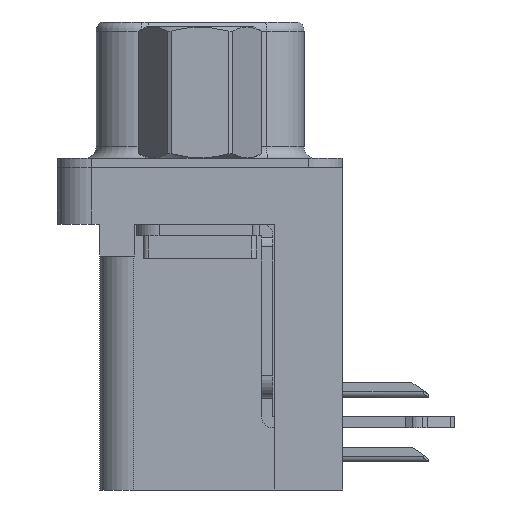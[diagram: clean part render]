
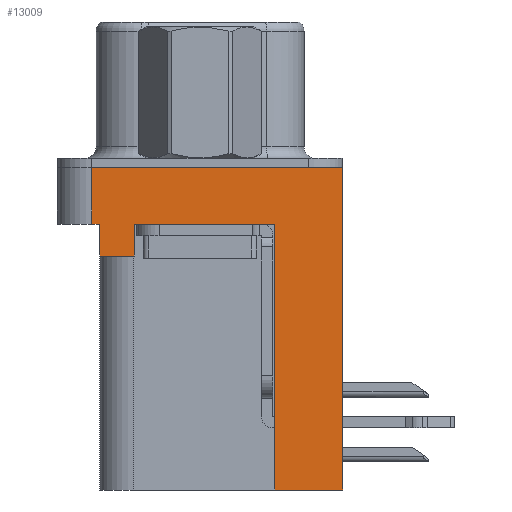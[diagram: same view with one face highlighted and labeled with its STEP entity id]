
A CAD part, left-side view. The second image highlights one B-rep face of the part: STEP entity #13009.
In plain terms, the highlighted planar face has unit normal (-1, 0, 0).
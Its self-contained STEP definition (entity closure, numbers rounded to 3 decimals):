
#144 = DIRECTION ( 'NONE',  ( 0., 1., 0. ) ) ;
#608 = CARTESIAN_POINT ( 'NONE',  ( -2.935, -6.275, -2.5 ) ) ;
#671 = VERTEX_POINT ( 'NONE', #20558 ) ;
#675 = VECTOR ( 'NONE', #144, 1000. ) ;
#1145 = CARTESIAN_POINT ( 'NONE',  ( -2.935, -6.275, 0. ) ) ;
#1560 = ORIENTED_EDGE ( 'NONE', *, *, #6238, .T. ) ;
#1581 = DIRECTION ( 'NONE',  ( 0., 0., 1. ) ) ;
#1715 = VERTEX_POINT ( 'NONE', #3816 ) ;
#1782 = CARTESIAN_POINT ( 'NONE',  ( -2.935, -6.275, -2.5 ) ) ;
#1913 = DIRECTION ( 'NONE',  ( 0., 0., 1. ) ) ;
#2252 = LINE ( 'NONE', #1782, #15737 ) ;
#2701 = EDGE_CURVE ( 'NONE', #4953, #7491, #7472, .T. ) ;
#2882 = VECTOR ( 'NONE', #22540, 1000. ) ;
#3191 = VERTEX_POINT ( 'NONE', #9280 ) ;
#3260 = DIRECTION ( 'NONE',  ( -1., 0., 0. ) ) ;
#3447 = DIRECTION ( 'NONE',  ( 0., 1., 0. ) ) ;
#3816 = CARTESIAN_POINT ( 'NONE',  ( -2.935, 2.895, -3.9 ) ) ;
#4017 = VECTOR ( 'NONE', #13824, 1000. ) ;
#4367 = VERTEX_POINT ( 'NONE', #1145 ) ;
#4953 = VERTEX_POINT ( 'NONE', #17877 ) ;
#5112 = FACE_OUTER_BOUND ( 'NONE', #14673, .T. ) ;
#5214 = LINE ( 'NONE', #7188, #12640 ) ;
#5245 = VERTEX_POINT ( 'NONE', #13289 ) ;
#5697 = ORIENTED_EDGE ( 'NONE', *, *, #7533, .F. ) ;
#6238 = EDGE_CURVE ( 'NONE', #671, #11153, #6294, .T. ) ;
#6294 = LINE ( 'NONE', #608, #4017 ) ;
#6390 = VECTOR ( 'NONE', #9056, 1000. ) ;
#6643 = LINE ( 'NONE', #15786, #23286 ) ;
#7016 = CARTESIAN_POINT ( 'NONE',  ( -2.935, 4.425, -2.5 ) ) ;
#7090 = CARTESIAN_POINT ( 'NONE',  ( -2.935, 4.425, -3.9 ) ) ;
#7188 = CARTESIAN_POINT ( 'NONE',  ( -2.935, -6.275, 0. ) ) ;
#7472 = LINE ( 'NONE', #15000, #2882 ) ;
#7491 = VERTEX_POINT ( 'NONE', #19983 ) ;
#7533 = EDGE_CURVE ( 'NONE', #3191, #7491, #6643, .T. ) ;
#7663 = ORIENTED_EDGE ( 'NONE', *, *, #13663, .F. ) ;
#7685 = EDGE_CURVE ( 'NONE', #671, #15482, #10814, .T. ) ;
#7707 = DIRECTION ( 'NONE',  ( 0., 0., 1. ) ) ;
#7721 = VERTEX_POINT ( 'NONE', #13651 ) ;
#7838 = ORIENTED_EDGE ( 'NONE', *, *, #11479, .T. ) ;
#9056 = DIRECTION ( 'NONE',  ( 0., 0., 1. ) ) ;
#9280 = CARTESIAN_POINT ( 'NONE',  ( -2.935, -3.295, -14.2 ) ) ;
#10090 = ORIENTED_EDGE ( 'NONE', *, *, #23882, .F. ) ;
#10347 = EDGE_CURVE ( 'NONE', #15482, #4367, #5214, .T. ) ;
#10777 = DIRECTION ( 'NONE',  ( 0., 0., 1. ) ) ;
#10814 = LINE ( 'NONE', #22573, #17804 ) ;
#10858 = DIRECTION ( 'NONE',  ( 0., -1., 0. ) ) ;
#11153 = VERTEX_POINT ( 'NONE', #7016 ) ;
#11235 = CARTESIAN_POINT ( 'NONE',  ( -2.935, 4.425, -3.9 ) ) ;
#11479 = EDGE_CURVE ( 'NONE', #1715, #4953, #24404, .T. ) ;
#11815 = EDGE_CURVE ( 'NONE', #5245, #11153, #12885, .T. ) ;
#12033 = ORIENTED_EDGE ( 'NONE', *, *, #11815, .F. ) ;
#12392 = ORIENTED_EDGE ( 'NONE', *, *, #23029, .T. ) ;
#12460 = AXIS2_PLACEMENT_3D ( 'NONE', #20199, #3260, #10777 ) ;
#12609 = VECTOR ( 'NONE', #3447, 1000. ) ;
#12639 = PLANE ( 'NONE',  #12460 ) ;
#12640 = VECTOR ( 'NONE', #10858, 1000. ) ;
#12885 = LINE ( 'NONE', #7090, #6390 ) ;
#13009 = ADVANCED_FACE ( 'NONE', ( #5112 ), #12639, .T. ) ;
#13107 = LINE ( 'NONE', #11235, #675 ) ;
#13240 = ORIENTED_EDGE ( 'NONE', *, *, #7685, .F. ) ;
#13289 = CARTESIAN_POINT ( 'NONE',  ( -2.935, 4.425, -3.9 ) ) ;
#13651 = CARTESIAN_POINT ( 'NONE',  ( -2.935, -6.275, -14.2 ) ) ;
#13663 = EDGE_CURVE ( 'NONE', #1715, #5245, #13107, .T. ) ;
#13824 = DIRECTION ( 'NONE',  ( 0., -1., 0. ) ) ;
#14673 = EDGE_LOOP ( 'NONE', ( #20952, #13240, #1560, #12033, #7663, #7838, #16852, #5697, #10090, #12392 ) ) ;
#14810 = CARTESIAN_POINT ( 'NONE',  ( -2.935, -3.295, -14.2 ) ) ;
#15000 = CARTESIAN_POINT ( 'NONE',  ( -2.935, -6.275, -2.5 ) ) ;
#15446 = VECTOR ( 'NONE', #1913, 1000. ) ;
#15482 = VERTEX_POINT ( 'NONE', #22474 ) ;
#15737 = VECTOR ( 'NONE', #7707, 1000. ) ;
#15786 = CARTESIAN_POINT ( 'NONE',  ( -2.935, -3.295, -14.2 ) ) ;
#16852 = ORIENTED_EDGE ( 'NONE', *, *, #2701, .T. ) ;
#17804 = VECTOR ( 'NONE', #1581, 1000. ) ;
#17877 = CARTESIAN_POINT ( 'NONE',  ( -2.935, 2.895, -2.5 ) ) ;
#19983 = CARTESIAN_POINT ( 'NONE',  ( -2.935, -3.295, -2.5 ) ) ;
#20109 = DIRECTION ( 'NONE',  ( 0., 0., 1. ) ) ;
#20199 = CARTESIAN_POINT ( 'NONE',  ( -2.935, -6.275, -2.5 ) ) ;
#20558 = CARTESIAN_POINT ( 'NONE',  ( -2.935, 4.775, -2.5 ) ) ;
#20952 = ORIENTED_EDGE ( 'NONE', *, *, #10347, .F. ) ;
#22468 = LINE ( 'NONE', #14810, #12609 ) ;
#22474 = CARTESIAN_POINT ( 'NONE',  ( -2.935, 4.775, 0. ) ) ;
#22540 = DIRECTION ( 'NONE',  ( 0., -1., 0. ) ) ;
#22573 = CARTESIAN_POINT ( 'NONE',  ( -2.935, 4.775, -2.5 ) ) ;
#23029 = EDGE_CURVE ( 'NONE', #7721, #4367, #2252, .T. ) ;
#23031 = CARTESIAN_POINT ( 'NONE',  ( -2.935, 2.895, -3.9 ) ) ;
#23286 = VECTOR ( 'NONE', #20109, 1000. ) ;
#23882 = EDGE_CURVE ( 'NONE', #7721, #3191, #22468, .T. ) ;
#24404 = LINE ( 'NONE', #23031, #15446 ) ;
